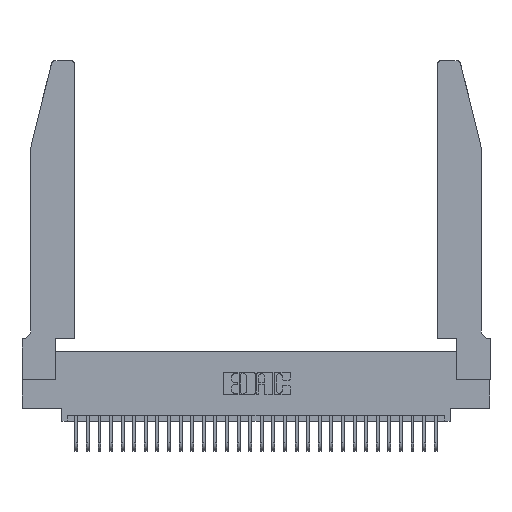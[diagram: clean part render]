
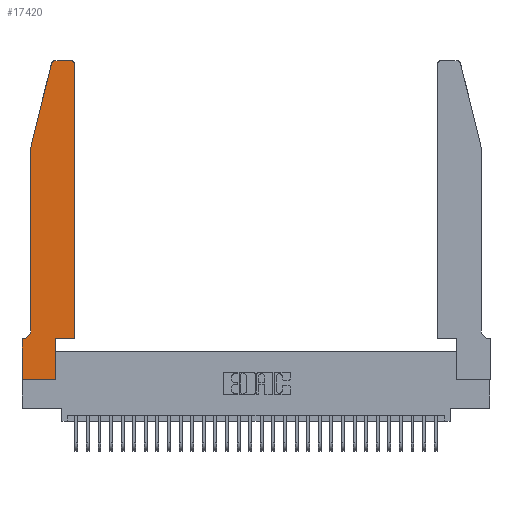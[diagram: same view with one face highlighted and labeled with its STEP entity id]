
A CAD part, top view. The second image highlights one B-rep face of the part: STEP entity #17420.
In plain terms, the highlighted planar face has unit normal (0, 0, 1).
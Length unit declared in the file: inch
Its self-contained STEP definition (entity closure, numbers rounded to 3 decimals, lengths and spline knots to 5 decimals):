
#129 = EDGE_CURVE ( 'NONE', #11565, #2923, #19550, .T. ) ;
#203 = CARTESIAN_POINT ( 'NONE',  ( 0.2605, 2.75, 0.37 ) ) ;
#505 = AXIS2_PLACEMENT_3D ( 'NONE', #2926, #3138, #30672 ) ;
#544 = LINE ( 'NONE', #6993, #20556 ) ;
#1165 = CARTESIAN_POINT ( 'NONE',  ( 0.4505, 2.72, 0.37 ) ) ;
#1630 = DIRECTION ( 'NONE',  ( -1., 0., 0. ) ) ;
#2297 = DIRECTION ( 'NONE',  ( -1., 0., 0. ) ) ;
#2923 = VERTEX_POINT ( 'NONE', #32921 ) ;
#2926 = CARTESIAN_POINT ( 'NONE',  ( 0.284, 2.72, 0.37 ) ) ;
#3138 = DIRECTION ( 'NONE',  ( 0., 0., 1. ) ) ;
#3209 = CARTESIAN_POINT ( 'NONE',  ( 0.4205, 2.75, 0.37 ) ) ;
#3307 = ORIENTED_EDGE ( 'NONE', *, *, #129, .T. ) ;
#3383 = ORIENTED_EDGE ( 'NONE', *, *, #15716, .T. ) ;
#3525 = CIRCLE ( 'NONE', #4178, 0.03 ) ;
#3777 = CARTESIAN_POINT ( 'NONE',  ( 0.0755, 0.35, 0.37 ) ) ;
#3812 = EDGE_CURVE ( 'NONE', #29660, #30609, #15811, .T. ) ;
#4041 = EDGE_CURVE ( 'NONE', #14357, #29660, #22982, .T. ) ;
#4178 = AXIS2_PLACEMENT_3D ( 'NONE', #19787, #14510, #22310 ) ;
#4395 = VECTOR ( 'NONE', #32304, 39.37008 ) ;
#4634 = CARTESIAN_POINT ( 'NONE',  ( 0.284, 2.75, 0.37 ) ) ;
#5447 = CARTESIAN_POINT ( 'NONE',  ( 0.0755, 2., 0.37 ) ) ;
#6514 = DIRECTION ( 'NONE',  ( 0., -1., 0. ) ) ;
#6628 = EDGE_CURVE ( 'NONE', #30609, #11565, #12064, .T. ) ;
#6993 = CARTESIAN_POINT ( 'NONE',  ( 0., 0., 0.37 ) ) ;
#7157 = ORIENTED_EDGE ( 'NONE', *, *, #4041, .T. ) ;
#7610 = CARTESIAN_POINT ( 'NONE',  ( 0., 0.35, 0.37 ) ) ;
#8203 = CARTESIAN_POINT ( 'NONE',  ( 0.0055, 0.35, 0.37 ) ) ;
#8638 = EDGE_CURVE ( 'NONE', #2923, #17206, #22655, .T. ) ;
#8993 = CARTESIAN_POINT ( 'NONE',  ( 0.0055, 0.42, 0.37 ) ) ;
#10625 = ORIENTED_EDGE ( 'NONE', *, *, #28959, .T. ) ;
#11018 = VECTOR ( 'NONE', #2297, 39.37008 ) ;
#11565 = VERTEX_POINT ( 'NONE', #5447 ) ;
#11843 = LINE ( 'NONE', #14123, #28107 ) ;
#12064 = LINE ( 'NONE', #26069, #24408 ) ;
#12706 = PLANE ( 'NONE',  #21932 ) ;
#12740 = DIRECTION ( 'NONE',  ( 0., 0., 1. ) ) ;
#13196 = ORIENTED_EDGE ( 'NONE', *, *, #6628, .T. ) ;
#13959 = LINE ( 'NONE', #14667, #23939 ) ;
#14123 = CARTESIAN_POINT ( 'NONE',  ( 0., 0., 0.37 ) ) ;
#14150 = DIRECTION ( 'NONE',  ( 0., -1., 0. ) ) ;
#14357 = VERTEX_POINT ( 'NONE', #3209 ) ;
#14488 = CARTESIAN_POINT ( 'NONE',  ( 0.4505, 0.35, 0.37 ) ) ;
#14510 = DIRECTION ( 'NONE',  ( 0., 0., 1. ) ) ;
#14667 = CARTESIAN_POINT ( 'NONE',  ( 0.4505, 0.35, 0.37 ) ) ;
#14725 = CARTESIAN_POINT ( 'NONE',  ( 0.4505, 0.35, 0.37 ) ) ;
#14762 = ORIENTED_EDGE ( 'NONE', *, *, #19623, .T. ) ;
#14780 = LINE ( 'NONE', #26611, #32332 ) ;
#15435 = ORIENTED_EDGE ( 'NONE', *, *, #8638, .T. ) ;
#15439 = EDGE_CURVE ( 'NONE', #24593, #24300, #14780, .T. ) ;
#15716 = EDGE_CURVE ( 'NONE', #24300, #31161, #13959, .T. ) ;
#15811 = CIRCLE ( 'NONE', #505, 0.03 ) ;
#17206 = VERTEX_POINT ( 'NONE', #8203 ) ;
#17420 = ADVANCED_FACE ( 'NONE', ( #17619 ), #12706, .T. ) ;
#17619 = FACE_OUTER_BOUND ( 'NONE', #24304, .T. ) ;
#19158 = ORIENTED_EDGE ( 'NONE', *, *, #15439, .T. ) ;
#19550 = LINE ( 'NONE', #22057, #31408 ) ;
#19623 = EDGE_CURVE ( 'NONE', #21764, #22818, #11843, .T. ) ;
#19698 = AXIS2_PLACEMENT_3D ( 'NONE', #8993, #29565, #1630 ) ;
#19787 = CARTESIAN_POINT ( 'NONE',  ( 0.4205, 2.72, 0.37 ) ) ;
#20556 = VECTOR ( 'NONE', #27376, 39.37008 ) ;
#21726 = CARTESIAN_POINT ( 'NONE',  ( 0.2865, 0., 0.37 ) ) ;
#21764 = VERTEX_POINT ( 'NONE', #31215 ) ;
#21932 = AXIS2_PLACEMENT_3D ( 'NONE', #7610, #12740, #30193 ) ;
#21960 = ORIENTED_EDGE ( 'NONE', *, *, #3812, .T. ) ;
#22000 = VERTEX_POINT ( 'NONE', #1165 ) ;
#22057 = CARTESIAN_POINT ( 'NONE',  ( 0.0755, 2., 0.37 ) ) ;
#22310 = DIRECTION ( 'NONE',  ( 1., 0., 0. ) ) ;
#22549 = EDGE_CURVE ( 'NONE', #17206, #21764, #25976, .T. ) ;
#22655 = CIRCLE ( 'NONE', #19698, 0.07 ) ;
#22818 = VERTEX_POINT ( 'NONE', #30846 ) ;
#22852 = CARTESIAN_POINT ( 'NONE',  ( 0.2865, 0.35, 0.37 ) ) ;
#22982 = LINE ( 'NONE', #203, #11018 ) ;
#23538 = ORIENTED_EDGE ( 'NONE', *, *, #28009, .T. ) ;
#23880 = DIRECTION ( 'NONE',  ( -1., 0., 0. ) ) ;
#23939 = VECTOR ( 'NONE', #25343, 39.37008 ) ;
#24300 = VERTEX_POINT ( 'NONE', #22852 ) ;
#24304 = EDGE_LOOP ( 'NONE', ( #7157, #21960, #13196, #3307, #15435, #27869, #14762, #28982, #19158, #3383, #23538, #10625 ) ) ;
#24408 = VECTOR ( 'NONE', #25861, 39.37008 ) ;
#24593 = VERTEX_POINT ( 'NONE', #21726 ) ;
#25343 = DIRECTION ( 'NONE',  ( 1., 0., 0. ) ) ;
#25861 = DIRECTION ( 'NONE',  ( -0.239, -0.971, 0. ) ) ;
#25933 = LINE ( 'NONE', #14488, #4395 ) ;
#25976 = LINE ( 'NONE', #3777, #29150 ) ;
#26069 = CARTESIAN_POINT ( 'NONE',  ( 0.0755, 2., 0.37 ) ) ;
#26611 = CARTESIAN_POINT ( 'NONE',  ( 0.2865, 0.35, 0.37 ) ) ;
#27376 = DIRECTION ( 'NONE',  ( 1., 0., 0. ) ) ;
#27869 = ORIENTED_EDGE ( 'NONE', *, *, #22549, .T. ) ;
#28009 = EDGE_CURVE ( 'NONE', #31161, #22000, #25933, .T. ) ;
#28107 = VECTOR ( 'NONE', #6514, 39.37008 ) ;
#28959 = EDGE_CURVE ( 'NONE', #22000, #14357, #3525, .T. ) ;
#28982 = ORIENTED_EDGE ( 'NONE', *, *, #31636, .T. ) ;
#29150 = VECTOR ( 'NONE', #23880, 39.37008 ) ;
#29565 = DIRECTION ( 'NONE',  ( 0., 0., -1. ) ) ;
#29660 = VERTEX_POINT ( 'NONE', #4634 ) ;
#30193 = DIRECTION ( 'NONE',  ( 1., 0., 0. ) ) ;
#30609 = VERTEX_POINT ( 'NONE', #32905 ) ;
#30672 = DIRECTION ( 'NONE',  ( 1., 0., 0. ) ) ;
#30846 = CARTESIAN_POINT ( 'NONE',  ( 0., 0., 0.37 ) ) ;
#31161 = VERTEX_POINT ( 'NONE', #14725 ) ;
#31215 = CARTESIAN_POINT ( 'NONE',  ( 0., 0.35, 0.37 ) ) ;
#31408 = VECTOR ( 'NONE', #14150, 39.37008 ) ;
#31475 = DIRECTION ( 'NONE',  ( 0., 1., 0. ) ) ;
#31636 = EDGE_CURVE ( 'NONE', #22818, #24593, #544, .T. ) ;
#32304 = DIRECTION ( 'NONE',  ( 0., 1., 0. ) ) ;
#32332 = VECTOR ( 'NONE', #31475, 39.37008 ) ;
#32905 = CARTESIAN_POINT ( 'NONE',  ( 0.25487, 2.72718, 0.37 ) ) ;
#32921 = CARTESIAN_POINT ( 'NONE',  ( 0.0755, 0.42, 0.37 ) ) ;
